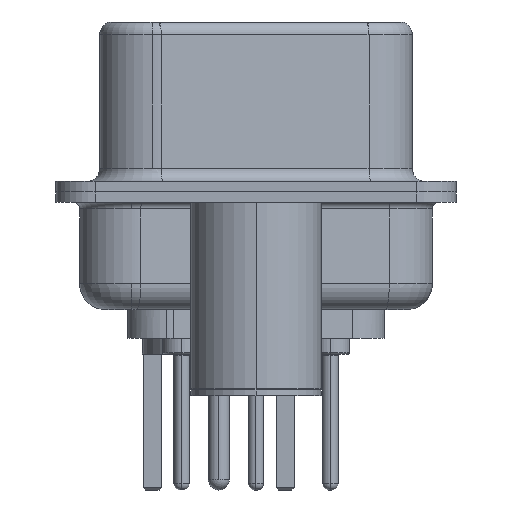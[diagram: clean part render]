
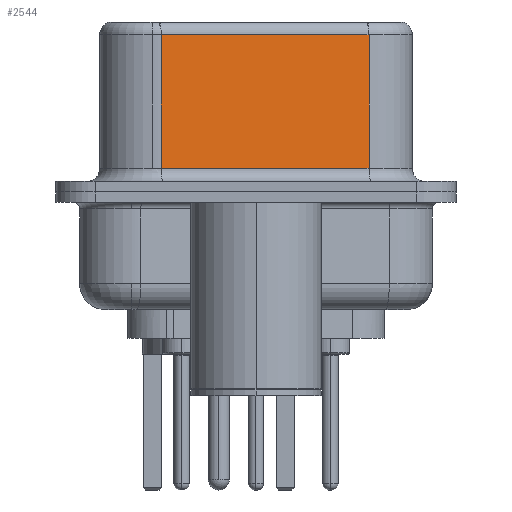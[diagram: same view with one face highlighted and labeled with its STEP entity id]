
A CAD part, left-side view. The second image highlights one B-rep face of the part: STEP entity #2544.
In plain terms, the highlighted planar face has unit normal (-0.985, -0.174, 0).
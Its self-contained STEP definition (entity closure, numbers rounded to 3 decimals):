
#830 = CARTESIAN_POINT ( 'NONE',  ( 3.73, 3.628, 6.02 ) ) ;
#2544 = ADVANCED_FACE ( 'NONE', ( #5369 ), #13364, .F. ) ;
#3568 = CARTESIAN_POINT ( 'NONE',  ( 5.132, -4.322, 0.9 ) ) ;
#3758 = VERTEX_POINT ( 'NONE', #830 ) ;
#3905 = AXIS2_PLACEMENT_3D ( 'NONE', #8439, #31208, #5769 ) ;
#3990 = DIRECTION ( 'NONE',  ( 0., 0., -1. ) ) ;
#4209 = ORIENTED_EDGE ( 'NONE', *, *, #14023, .T. ) ;
#4217 = DIRECTION ( 'NONE',  ( -0.174, 0.985, 0. ) ) ;
#5369 = FACE_OUTER_BOUND ( 'NONE', #9300, .T. ) ;
#5682 = CARTESIAN_POINT ( 'NONE',  ( 5.132, -4.322, 6.02 ) ) ;
#5769 = DIRECTION ( 'NONE',  ( -0.174, 0.985, 0. ) ) ;
#5886 = ORIENTED_EDGE ( 'NONE', *, *, #10375, .F. ) ;
#6100 = VECTOR ( 'NONE', #4217, 1000. ) ;
#7751 = LINE ( 'NONE', #19092, #10913 ) ;
#8439 = CARTESIAN_POINT ( 'NONE',  ( 5.132, -4.322, 6.52 ) ) ;
#9300 = EDGE_LOOP ( 'NONE', ( #5886, #11540, #29693, #4209 ) ) ;
#10375 = EDGE_CURVE ( 'NONE', #12079, #32422, #7751, .T. ) ;
#10913 = VECTOR ( 'NONE', #3990, 1000. ) ;
#11540 = ORIENTED_EDGE ( 'NONE', *, *, #30843, .T. ) ;
#12079 = VERTEX_POINT ( 'NONE', #20494 ) ;
#12084 = VECTOR ( 'NONE', #26245, 1000. ) ;
#13364 = PLANE ( 'NONE',  #3905 ) ;
#14023 = EDGE_CURVE ( 'NONE', #15879, #32422, #14833, .T. ) ;
#14331 = CARTESIAN_POINT ( 'NONE',  ( 3.73, 3.628, 0.9 ) ) ;
#14833 = LINE ( 'NONE', #28598, #12084 ) ;
#15879 = VERTEX_POINT ( 'NONE', #14331 ) ;
#19092 = CARTESIAN_POINT ( 'NONE',  ( 5.132, -4.322, 6.52 ) ) ;
#20494 = CARTESIAN_POINT ( 'NONE',  ( 5.132, -4.322, 6.02 ) ) ;
#20997 = DIRECTION ( 'NONE',  ( 0., 0., -1. ) ) ;
#25568 = VECTOR ( 'NONE', #20997, 1000. ) ;
#26245 = DIRECTION ( 'NONE',  ( 0.174, -0.985, 0. ) ) ;
#27423 = LINE ( 'NONE', #5682, #6100 ) ;
#28598 = CARTESIAN_POINT ( 'NONE',  ( 5.132, -4.322, 0.9 ) ) ;
#28662 = EDGE_CURVE ( 'NONE', #3758, #15879, #32347, .T. ) ;
#29693 = ORIENTED_EDGE ( 'NONE', *, *, #28662, .T. ) ;
#30843 = EDGE_CURVE ( 'NONE', #12079, #3758, #27423, .T. ) ;
#30922 = CARTESIAN_POINT ( 'NONE',  ( 3.73, 3.628, 6.52 ) ) ;
#31208 = DIRECTION ( 'NONE',  ( 0.985, 0.174, 0. ) ) ;
#32347 = LINE ( 'NONE', #30922, #25568 ) ;
#32422 = VERTEX_POINT ( 'NONE', #3568 ) ;
